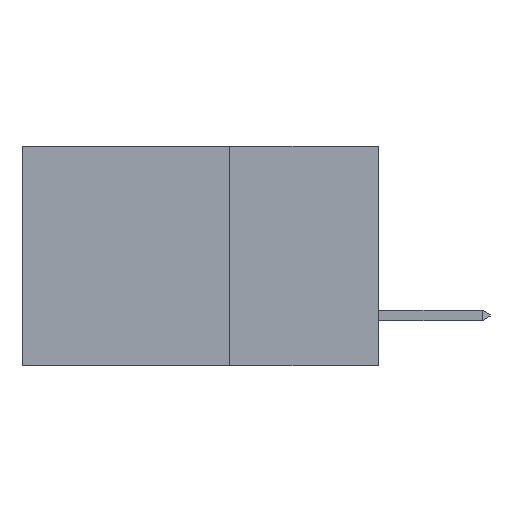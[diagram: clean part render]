
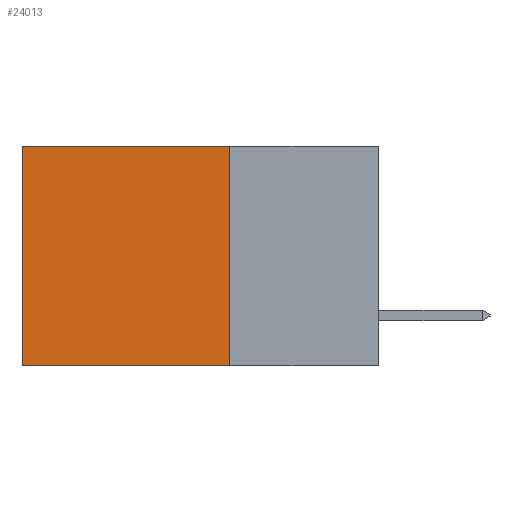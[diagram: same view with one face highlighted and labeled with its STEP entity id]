
A CAD part, left-side view. The second image highlights one B-rep face of the part: STEP entity #24013.
In plain terms, the highlighted planar face has unit normal (-1, 0, 0).
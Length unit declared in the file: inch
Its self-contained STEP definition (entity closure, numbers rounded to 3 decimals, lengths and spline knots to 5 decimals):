
#778 = CARTESIAN_POINT ( 'NONE',  ( 0.298, 0.25, 0. ) ) ;
#1105 = CARTESIAN_POINT ( 'NONE',  ( 0.298, 0.25, 0. ) ) ;
#2280 = ORIENTED_EDGE ( 'NONE', *, *, #2445, .T. ) ;
#2445 = EDGE_CURVE ( 'NONE', #13478, #26954, #19988, .T. ) ;
#2708 = DIRECTION ( 'NONE',  ( 0., 1., 0. ) ) ;
#3400 = PLANE ( 'NONE',  #20853 ) ;
#3607 = VERTEX_POINT ( 'NONE', #26679 ) ;
#3906 = DIRECTION ( 'NONE',  ( 0., 1., 0. ) ) ;
#4090 = CARTESIAN_POINT ( 'NONE',  ( 0.298, 0.6, -0.37 ) ) ;
#4560 = LINE ( 'NONE', #778, #10522 ) ;
#5295 = EDGE_CURVE ( 'NONE', #14491, #26954, #20754, .T. ) ;
#7877 = DIRECTION ( 'NONE',  ( 1., 0., 0. ) ) ;
#8553 = FACE_OUTER_BOUND ( 'NONE', #22885, .T. ) ;
#9343 = CARTESIAN_POINT ( 'NONE',  ( 0.298, 0.6, 0. ) ) ;
#10522 = VECTOR ( 'NONE', #25225, 39.37008 ) ;
#11558 = ORIENTED_EDGE ( 'NONE', *, *, #17098, .T. ) ;
#11801 = ORIENTED_EDGE ( 'NONE', *, *, #5295, .F. ) ;
#11862 = ORIENTED_EDGE ( 'NONE', *, *, #20937, .F. ) ;
#12033 = VECTOR ( 'NONE', #28803, 39.37008 ) ;
#13478 = VERTEX_POINT ( 'NONE', #21863 ) ;
#13851 = CARTESIAN_POINT ( 'NONE',  ( 0.298, 0.25, 0. ) ) ;
#14491 = VERTEX_POINT ( 'NONE', #21317 ) ;
#17098 = EDGE_CURVE ( 'NONE', #3607, #13478, #27701, .T. ) ;
#19988 = LINE ( 'NONE', #9343, #12033 ) ;
#20754 = LINE ( 'NONE', #28227, #25945 ) ;
#20853 = AXIS2_PLACEMENT_3D ( 'NONE', #1105, #7877, #23424 ) ;
#20937 = EDGE_CURVE ( 'NONE', #3607, #14491, #4560, .T. ) ;
#21317 = CARTESIAN_POINT ( 'NONE',  ( 0.298, 0.25, -0.37 ) ) ;
#21863 = CARTESIAN_POINT ( 'NONE',  ( 0.298, 0.6, 0. ) ) ;
#22885 = EDGE_LOOP ( 'NONE', ( #2280, #11801, #11862, #11558 ) ) ;
#23424 = DIRECTION ( 'NONE',  ( 0., 0., -1. ) ) ;
#24013 = ADVANCED_FACE ( 'NONE', ( #8553 ), #3400, .F. ) ;
#25225 = DIRECTION ( 'NONE',  ( 0., 0., -1. ) ) ;
#25945 = VECTOR ( 'NONE', #3906, 39.37008 ) ;
#26330 = VECTOR ( 'NONE', #2708, 39.37008 ) ;
#26679 = CARTESIAN_POINT ( 'NONE',  ( 0.298, 0.25, 0. ) ) ;
#26954 = VERTEX_POINT ( 'NONE', #4090 ) ;
#27701 = LINE ( 'NONE', #13851, #26330 ) ;
#28227 = CARTESIAN_POINT ( 'NONE',  ( 0.298, 0.25, -0.37 ) ) ;
#28803 = DIRECTION ( 'NONE',  ( 0., 0., -1. ) ) ;
